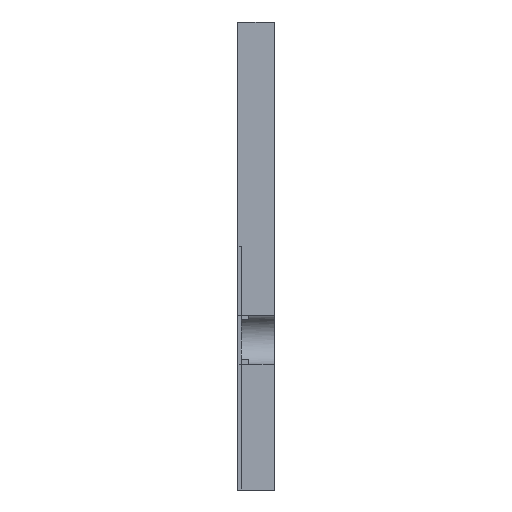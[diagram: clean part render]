
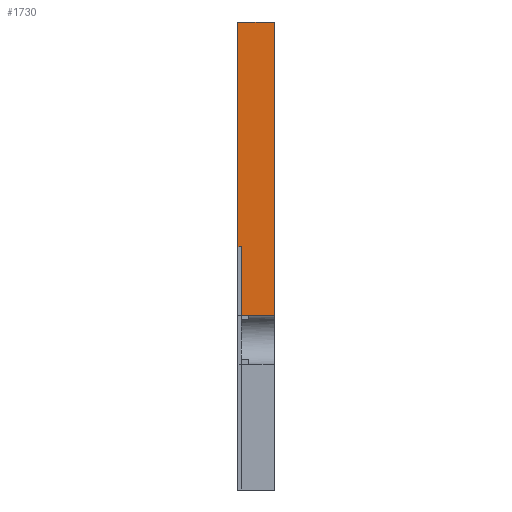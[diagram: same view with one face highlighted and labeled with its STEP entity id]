
A CAD part, left-side view. The second image highlights one B-rep face of the part: STEP entity #1730.
In plain terms, the highlighted planar face has unit normal (-1, 0, 0).
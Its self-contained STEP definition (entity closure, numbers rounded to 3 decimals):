
#51 = PLANE ( 'NONE',  #68 ) ;
#53 = CARTESIAN_POINT ( 'NONE',  ( 0., -0.533, -30.931 ) ) ;
#68 = AXIS2_PLACEMENT_3D ( 'NONE', #1106, #342, #1403 ) ;
#89 = LINE ( 'NONE', #53, #1946 ) ;
#201 = VECTOR ( 'NONE', #681, 1000. ) ;
#205 = VERTEX_POINT ( 'NONE', #632 ) ;
#207 = DIRECTION ( 'NONE',  ( 0., 1., 0. ) ) ;
#277 = CARTESIAN_POINT ( 'NONE',  ( 0., -5., -40.361 ) ) ;
#311 = VERTEX_POINT ( 'NONE', #1069 ) ;
#314 = EDGE_CURVE ( 'NONE', #523, #205, #1450, .T. ) ;
#318 = VECTOR ( 'NONE', #1154, 1000. ) ;
#339 = CARTESIAN_POINT ( 'NONE',  ( 0., -0.533, -30.931 ) ) ;
#342 = DIRECTION ( 'NONE',  ( 1., 0., 0. ) ) ;
#368 = EDGE_CURVE ( 'NONE', #205, #699, #1360, .T. ) ;
#376 = VERTEX_POINT ( 'NONE', #1794 ) ;
#499 = CARTESIAN_POINT ( 'NONE',  ( 0., -5., 0. ) ) ;
#523 = VERTEX_POINT ( 'NONE', #776 ) ;
#595 = DIRECTION ( 'NONE',  ( 0., 0., 1. ) ) ;
#632 = CARTESIAN_POINT ( 'NONE',  ( 0., -0.533, -40.361 ) ) ;
#681 = DIRECTION ( 'NONE',  ( 0., 0., -1. ) ) ;
#686 = CARTESIAN_POINT ( 'NONE',  ( 0., -5., 0. ) ) ;
#696 = ORIENTED_EDGE ( 'NONE', *, *, #314, .F. ) ;
#698 = FACE_OUTER_BOUND ( 'NONE', #1490, .T. ) ;
#699 = VERTEX_POINT ( 'NONE', #339 ) ;
#719 = VERTEX_POINT ( 'NONE', #499 ) ;
#734 = DIRECTION ( 'NONE',  ( 0., 1., 0. ) ) ;
#751 = CARTESIAN_POINT ( 'NONE',  ( 0., 0., 0. ) ) ;
#776 = CARTESIAN_POINT ( 'NONE',  ( 0., -5., -40.361 ) ) ;
#854 = ORIENTED_EDGE ( 'NONE', *, *, #1491, .T. ) ;
#1013 = VECTOR ( 'NONE', #595, 1000. ) ;
#1021 = EDGE_CURVE ( 'NONE', #719, #523, #1361, .T. ) ;
#1061 = VECTOR ( 'NONE', #734, 1000. ) ;
#1069 = CARTESIAN_POINT ( 'NONE',  ( 0., 0., -30.931 ) ) ;
#1095 = ORIENTED_EDGE ( 'NONE', *, *, #1273, .T. ) ;
#1106 = CARTESIAN_POINT ( 'NONE',  ( 0., -5., 0. ) ) ;
#1154 = DIRECTION ( 'NONE',  ( 0., 1., 0. ) ) ;
#1224 = ORIENTED_EDGE ( 'NONE', *, *, #368, .F. ) ;
#1273 = EDGE_CURVE ( 'NONE', #376, #311, #1283, .T. ) ;
#1283 = LINE ( 'NONE', #751, #1675 ) ;
#1329 = EDGE_CURVE ( 'NONE', #699, #311, #89, .T. ) ;
#1360 = LINE ( 'NONE', #1644, #1013 ) ;
#1361 = LINE ( 'NONE', #1575, #201 ) ;
#1403 = DIRECTION ( 'NONE',  ( 0., 0., -1. ) ) ;
#1437 = ORIENTED_EDGE ( 'NONE', *, *, #1329, .F. ) ;
#1450 = LINE ( 'NONE', #277, #1061 ) ;
#1490 = EDGE_LOOP ( 'NONE', ( #1095, #1437, #1224, #696, #1942, #854 ) ) ;
#1491 = EDGE_CURVE ( 'NONE', #719, #376, #1928, .T. ) ;
#1575 = CARTESIAN_POINT ( 'NONE',  ( 0., -5., 0. ) ) ;
#1644 = CARTESIAN_POINT ( 'NONE',  ( 0., -0.533, -30.931 ) ) ;
#1646 = DIRECTION ( 'NONE',  ( 0., 0., -1. ) ) ;
#1675 = VECTOR ( 'NONE', #1646, 1000. ) ;
#1730 = ADVANCED_FACE ( 'NONE', ( #698 ), #51, .F. ) ;
#1794 = CARTESIAN_POINT ( 'NONE',  ( 0., 0., 0. ) ) ;
#1928 = LINE ( 'NONE', #686, #318 ) ;
#1942 = ORIENTED_EDGE ( 'NONE', *, *, #1021, .F. ) ;
#1946 = VECTOR ( 'NONE', #207, 1000. ) ;
